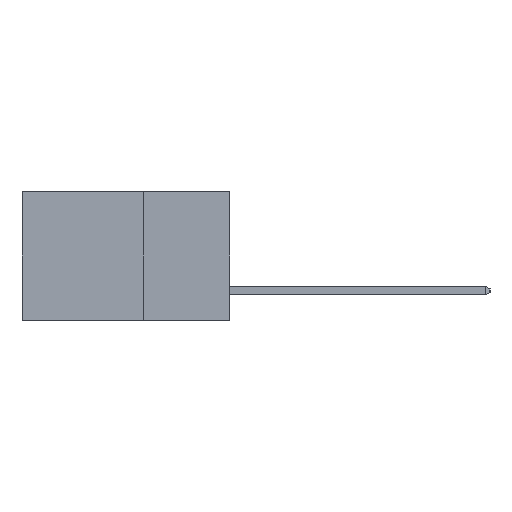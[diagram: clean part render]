
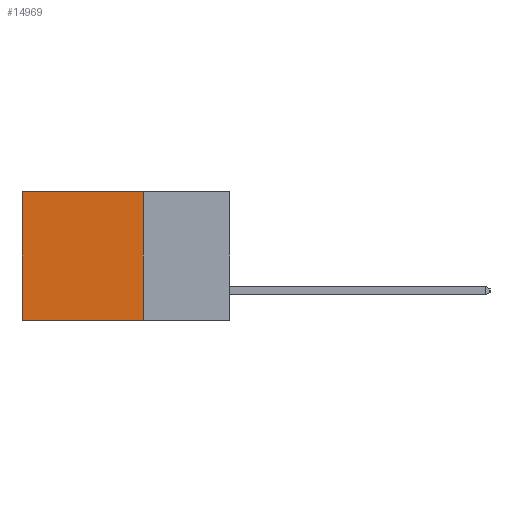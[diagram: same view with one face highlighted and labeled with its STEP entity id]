
A CAD part, left-side view. The second image highlights one B-rep face of the part: STEP entity #14969.
In plain terms, the highlighted planar face has unit normal (-1, 0, 0).
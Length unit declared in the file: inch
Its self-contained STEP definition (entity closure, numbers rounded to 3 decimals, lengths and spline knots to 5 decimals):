
#213 = VECTOR ( 'NONE', #16058, 39.37008 ) ;
#439 = VERTEX_POINT ( 'NONE', #8017 ) ;
#606 = EDGE_LOOP ( 'NONE', ( #661, #16747, #3625, #4611 ) ) ;
#661 = ORIENTED_EDGE ( 'NONE', *, *, #15422, .T. ) ;
#1542 = LINE ( 'NONE', #9639, #8448 ) ;
#1877 = LINE ( 'NONE', #12179, #8785 ) ;
#2409 = CARTESIAN_POINT ( 'NONE',  ( 0.298, 0.25, 0. ) ) ;
#2478 = EDGE_CURVE ( 'NONE', #7192, #439, #3889, .T. ) ;
#2521 = DIRECTION ( 'NONE',  ( 0., 0., -1. ) ) ;
#3238 = FACE_OUTER_BOUND ( 'NONE', #606, .T. ) ;
#3625 = ORIENTED_EDGE ( 'NONE', *, *, #4113, .F. ) ;
#3889 = LINE ( 'NONE', #17464, #213 ) ;
#4113 = EDGE_CURVE ( 'NONE', #6991, #7192, #1877, .T. ) ;
#4611 = ORIENTED_EDGE ( 'NONE', *, *, #6300, .T. ) ;
#4994 = DIRECTION ( 'NONE',  ( 0., 0., -1. ) ) ;
#6300 = EDGE_CURVE ( 'NONE', #6991, #16092, #1542, .T. ) ;
#6991 = VERTEX_POINT ( 'NONE', #2409 ) ;
#7192 = VERTEX_POINT ( 'NONE', #13742 ) ;
#7975 = VECTOR ( 'NONE', #13135, 39.37008 ) ;
#8017 = CARTESIAN_POINT ( 'NONE',  ( 0.298, 0.6, -0.37 ) ) ;
#8378 = LINE ( 'NONE', #11794, #7975 ) ;
#8448 = VECTOR ( 'NONE', #15166, 39.37008 ) ;
#8785 = VECTOR ( 'NONE', #4994, 39.37008 ) ;
#9099 = CARTESIAN_POINT ( 'NONE',  ( 0.298, 0.6, 0. ) ) ;
#9639 = CARTESIAN_POINT ( 'NONE',  ( 0.298, 0.25, 0. ) ) ;
#10780 = DIRECTION ( 'NONE',  ( 1., 0., 0. ) ) ;
#11794 = CARTESIAN_POINT ( 'NONE',  ( 0.298, 0.6, 0. ) ) ;
#12103 = CARTESIAN_POINT ( 'NONE',  ( 0.298, 0.25, 0. ) ) ;
#12179 = CARTESIAN_POINT ( 'NONE',  ( 0.298, 0.25, 0. ) ) ;
#13135 = DIRECTION ( 'NONE',  ( 0., 0., -1. ) ) ;
#13742 = CARTESIAN_POINT ( 'NONE',  ( 0.298, 0.25, -0.37 ) ) ;
#14771 = AXIS2_PLACEMENT_3D ( 'NONE', #12103, #10780, #2521 ) ;
#14969 = ADVANCED_FACE ( 'NONE', ( #3238 ), #17522, .F. ) ;
#15166 = DIRECTION ( 'NONE',  ( 0., 1., 0. ) ) ;
#15422 = EDGE_CURVE ( 'NONE', #16092, #439, #8378, .T. ) ;
#16058 = DIRECTION ( 'NONE',  ( 0., 1., 0. ) ) ;
#16092 = VERTEX_POINT ( 'NONE', #9099 ) ;
#16747 = ORIENTED_EDGE ( 'NONE', *, *, #2478, .F. ) ;
#17464 = CARTESIAN_POINT ( 'NONE',  ( 0.298, 0.25, -0.37 ) ) ;
#17522 = PLANE ( 'NONE',  #14771 ) ;
